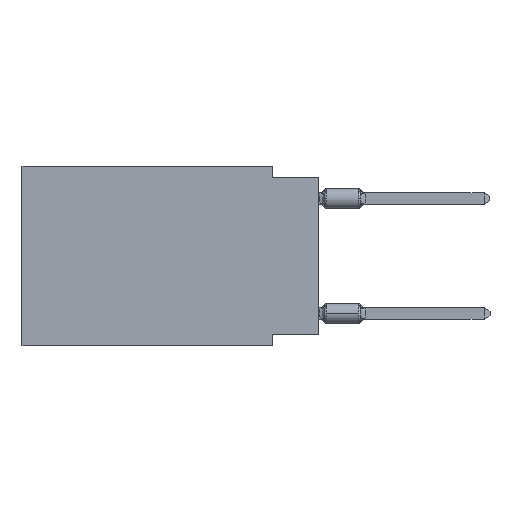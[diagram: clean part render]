
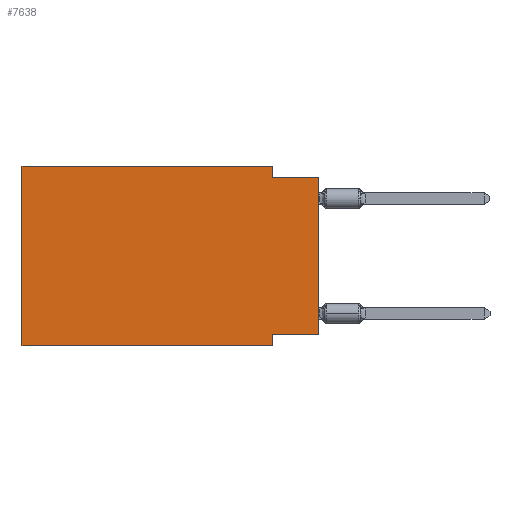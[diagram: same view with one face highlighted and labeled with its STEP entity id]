
A CAD part, left-side view. The second image highlights one B-rep face of the part: STEP entity #7638.
In plain terms, the highlighted planar face has unit normal (-1, 0, 0).
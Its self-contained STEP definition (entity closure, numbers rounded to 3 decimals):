
#91 = VERTEX_POINT ( 'NONE', #12276 ) ;
#258 = EDGE_CURVE ( 'NONE', #12129, #16606, #4445, .T. ) ;
#847 = EDGE_CURVE ( 'NONE', #10481, #12206, #18979, .T. ) ;
#969 = DIRECTION ( 'NONE',  ( 0., 0., 1. ) ) ;
#1108 = CARTESIAN_POINT ( 'NONE',  ( 0., 2.54, -9.906 ) ) ;
#1636 = CARTESIAN_POINT ( 'NONE',  ( 0., 16.383, 0. ) ) ;
#2024 = VECTOR ( 'NONE', #16820, 1000. ) ;
#2686 = LINE ( 'NONE', #16760, #9360 ) ;
#3058 = LINE ( 'NONE', #15394, #12615 ) ;
#3186 = ORIENTED_EDGE ( 'NONE', *, *, #8700, .F. ) ;
#4384 = ORIENTED_EDGE ( 'NONE', *, *, #9291, .F. ) ;
#4445 = LINE ( 'NONE', #1108, #12979 ) ;
#4465 = CARTESIAN_POINT ( 'NONE',  ( 0., 16.383, -9.906 ) ) ;
#4477 = EDGE_CURVE ( 'NONE', #11912, #91, #22147, .T. ) ;
#5429 = VERTEX_POINT ( 'NONE', #4465 ) ;
#5515 = ORIENTED_EDGE ( 'NONE', *, *, #7548, .F. ) ;
#6085 = CARTESIAN_POINT ( 'NONE',  ( 0., 0., -9.271 ) ) ;
#6086 = EDGE_LOOP ( 'NONE', ( #14645, #4384, #20634, #22029, #5515, #13232, #22014, #3186 ) ) ;
#6159 = VECTOR ( 'NONE', #13387, 1000. ) ;
#6422 = AXIS2_PLACEMENT_3D ( 'NONE', #1636, #22478, #10593 ) ;
#6600 = DIRECTION ( 'NONE',  ( 0., -1., 0. ) ) ;
#7548 = EDGE_CURVE ( 'NONE', #5429, #11912, #2686, .T. ) ;
#7638 = ADVANCED_FACE ( 'NONE', ( #17427 ), #17536, .F. ) ;
#7695 = CARTESIAN_POINT ( 'NONE',  ( 0., 0., -9.271 ) ) ;
#8117 = DIRECTION ( 'NONE',  ( 0., 0., -1. ) ) ;
#8700 = EDGE_CURVE ( 'NONE', #10481, #12129, #11725, .T. ) ;
#9291 = EDGE_CURVE ( 'NONE', #13134, #12206, #3058, .T. ) ;
#9360 = VECTOR ( 'NONE', #969, 1000. ) ;
#9416 = CARTESIAN_POINT ( 'NONE',  ( 0., 2.54, -9.906 ) ) ;
#9805 = CARTESIAN_POINT ( 'NONE',  ( 0., 16.383, 0. ) ) ;
#10481 = VERTEX_POINT ( 'NONE', #7695 ) ;
#10527 = CARTESIAN_POINT ( 'NONE',  ( 0., 0., 0. ) ) ;
#10593 = DIRECTION ( 'NONE',  ( 0., 0., -1. ) ) ;
#11090 = VECTOR ( 'NONE', #22639, 1000. ) ;
#11725 = LINE ( 'NONE', #6085, #2024 ) ;
#11912 = VERTEX_POINT ( 'NONE', #17738 ) ;
#12129 = VERTEX_POINT ( 'NONE', #18882 ) ;
#12130 = CARTESIAN_POINT ( 'NONE',  ( 0., 0., -0.635 ) ) ;
#12139 = CARTESIAN_POINT ( 'NONE',  ( 0., 16.383, -9.906 ) ) ;
#12206 = VERTEX_POINT ( 'NONE', #12130 ) ;
#12276 = CARTESIAN_POINT ( 'NONE',  ( 0., 2.54, 0. ) ) ;
#12615 = VECTOR ( 'NONE', #22408, 1000. ) ;
#12979 = VECTOR ( 'NONE', #8117, 1000. ) ;
#13134 = VERTEX_POINT ( 'NONE', #16788 ) ;
#13232 = ORIENTED_EDGE ( 'NONE', *, *, #21765, .T. ) ;
#13387 = DIRECTION ( 'NONE',  ( 0., -1., 0. ) ) ;
#14645 = ORIENTED_EDGE ( 'NONE', *, *, #847, .T. ) ;
#15394 = CARTESIAN_POINT ( 'NONE',  ( 0., 0., -0.635 ) ) ;
#16606 = VERTEX_POINT ( 'NONE', #9416 ) ;
#16760 = CARTESIAN_POINT ( 'NONE',  ( 0., 16.383, 0. ) ) ;
#16788 = CARTESIAN_POINT ( 'NONE',  ( 0., 2.54, -0.635 ) ) ;
#16820 = DIRECTION ( 'NONE',  ( 0., 1., 0. ) ) ;
#17427 = FACE_OUTER_BOUND ( 'NONE', #6086, .T. ) ;
#17536 = PLANE ( 'NONE',  #6422 ) ;
#17543 = LINE ( 'NONE', #20990, #21600 ) ;
#17738 = CARTESIAN_POINT ( 'NONE',  ( 0., 16.383, 0. ) ) ;
#17858 = VECTOR ( 'NONE', #6600, 1000. ) ;
#18882 = CARTESIAN_POINT ( 'NONE',  ( 0., 2.54, -9.271 ) ) ;
#18979 = LINE ( 'NONE', #10527, #11090 ) ;
#20497 = EDGE_CURVE ( 'NONE', #91, #13134, #17543, .T. ) ;
#20634 = ORIENTED_EDGE ( 'NONE', *, *, #20497, .F. ) ;
#20794 = LINE ( 'NONE', #12139, #17858 ) ;
#20990 = CARTESIAN_POINT ( 'NONE',  ( 0., 2.54, 0. ) ) ;
#21215 = DIRECTION ( 'NONE',  ( 0., 0., -1. ) ) ;
#21600 = VECTOR ( 'NONE', #21215, 1000. ) ;
#21765 = EDGE_CURVE ( 'NONE', #5429, #16606, #20794, .T. ) ;
#22014 = ORIENTED_EDGE ( 'NONE', *, *, #258, .F. ) ;
#22029 = ORIENTED_EDGE ( 'NONE', *, *, #4477, .F. ) ;
#22147 = LINE ( 'NONE', #9805, #6159 ) ;
#22408 = DIRECTION ( 'NONE',  ( 0., -1., 0. ) ) ;
#22478 = DIRECTION ( 'NONE',  ( 1., 0., 0. ) ) ;
#22639 = DIRECTION ( 'NONE',  ( 0., 0., 1. ) ) ;
